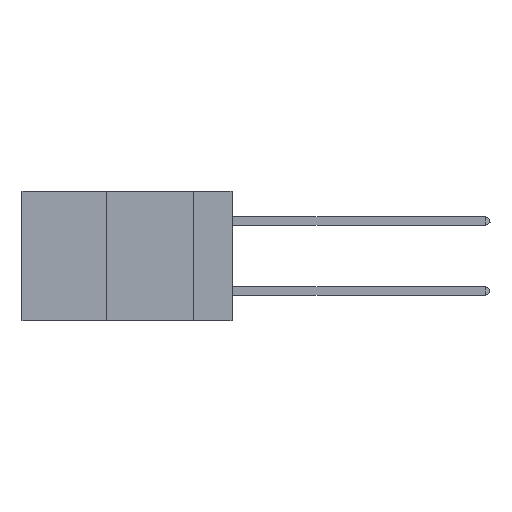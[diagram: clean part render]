
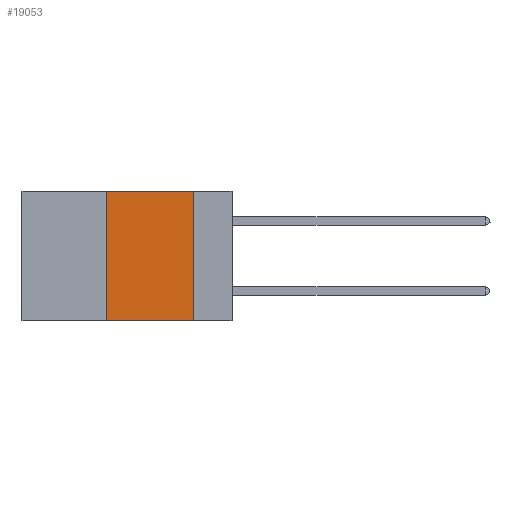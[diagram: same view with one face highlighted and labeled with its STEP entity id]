
A CAD part, left-side view. The second image highlights one B-rep face of the part: STEP entity #19053.
In plain terms, the highlighted planar face has unit normal (-1, 0, 0).
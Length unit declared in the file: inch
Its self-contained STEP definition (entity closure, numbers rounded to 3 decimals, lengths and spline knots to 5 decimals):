
#214 = CARTESIAN_POINT ( 'NONE',  ( 0., 0.36, -0.37 ) ) ;
#426 = VERTEX_POINT ( 'NONE', #7600 ) ;
#1519 = VECTOR ( 'NONE', #22598, 39.37008 ) ;
#2590 = EDGE_CURVE ( 'NONE', #17932, #22854, #5677, .T. ) ;
#3199 = DIRECTION ( 'NONE',  ( 0., -1., 0. ) ) ;
#3626 = ORIENTED_EDGE ( 'NONE', *, *, #8620, .T. ) ;
#4237 = VECTOR ( 'NONE', #3199, 39.37008 ) ;
#5677 = LINE ( 'NONE', #19172, #14928 ) ;
#5869 = VECTOR ( 'NONE', #19999, 39.37008 ) ;
#5945 = DIRECTION ( 'NONE',  ( 0., 0., -1. ) ) ;
#7600 = CARTESIAN_POINT ( 'NONE',  ( 0., 0.36, 0. ) ) ;
#7700 = DIRECTION ( 'NONE',  ( 1., 0., 0. ) ) ;
#8551 = ORIENTED_EDGE ( 'NONE', *, *, #19676, .F. ) ;
#8620 = EDGE_CURVE ( 'NONE', #15897, #22854, #12140, .T. ) ;
#10102 = ORIENTED_EDGE ( 'NONE', *, *, #16294, .F. ) ;
#12140 = LINE ( 'NONE', #15414, #1519 ) ;
#13841 = LINE ( 'NONE', #15591, #4237 ) ;
#14727 = PLANE ( 'NONE',  #21435 ) ;
#14928 = VECTOR ( 'NONE', #21519, 39.37008 ) ;
#15414 = CARTESIAN_POINT ( 'NONE',  ( 0., 0.6, -0.37 ) ) ;
#15591 = CARTESIAN_POINT ( 'NONE',  ( 0., 0.6, 0. ) ) ;
#15897 = VERTEX_POINT ( 'NONE', #214 ) ;
#16294 = EDGE_CURVE ( 'NONE', #15897, #426, #18110, .T. ) ;
#16849 = FACE_OUTER_BOUND ( 'NONE', #18733, .T. ) ;
#17932 = VERTEX_POINT ( 'NONE', #17967 ) ;
#17967 = CARTESIAN_POINT ( 'NONE',  ( 0., 0.11, 0. ) ) ;
#18110 = LINE ( 'NONE', #19653, #5869 ) ;
#18164 = ORIENTED_EDGE ( 'NONE', *, *, #2590, .F. ) ;
#18733 = EDGE_LOOP ( 'NONE', ( #18164, #8551, #10102, #3626 ) ) ;
#18878 = CARTESIAN_POINT ( 'NONE',  ( 0., 0.11, -0.37 ) ) ;
#19053 = ADVANCED_FACE ( 'NONE', ( #16849 ), #14727, .F. ) ;
#19172 = CARTESIAN_POINT ( 'NONE',  ( 0., 0.11, 0. ) ) ;
#19653 = CARTESIAN_POINT ( 'NONE',  ( 0., 0.36, 0. ) ) ;
#19676 = EDGE_CURVE ( 'NONE', #426, #17932, #13841, .T. ) ;
#19999 = DIRECTION ( 'NONE',  ( 0., 0., 1. ) ) ;
#21435 = AXIS2_PLACEMENT_3D ( 'NONE', #21903, #7700, #5945 ) ;
#21519 = DIRECTION ( 'NONE',  ( 0., 0., -1. ) ) ;
#21903 = CARTESIAN_POINT ( 'NONE',  ( 0., 0.6, 0. ) ) ;
#22598 = DIRECTION ( 'NONE',  ( 0., -1., 0. ) ) ;
#22854 = VERTEX_POINT ( 'NONE', #18878 ) ;
